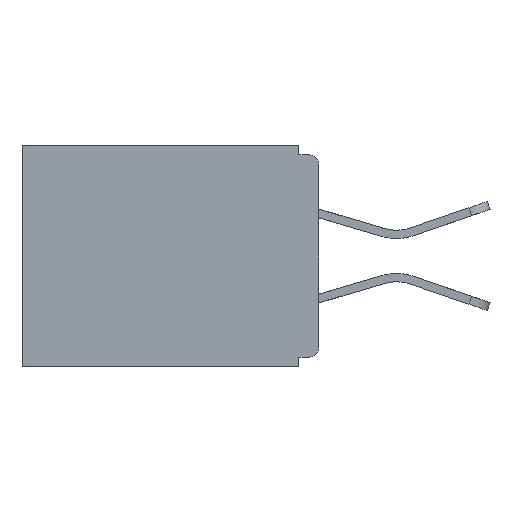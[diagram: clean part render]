
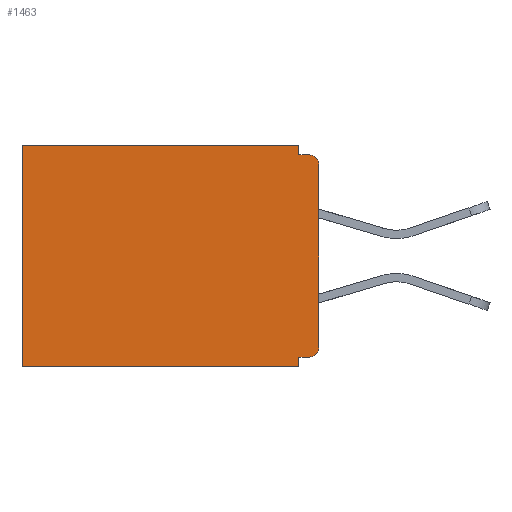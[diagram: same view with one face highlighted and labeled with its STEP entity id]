
A CAD part, left-side view. The second image highlights one B-rep face of the part: STEP entity #1463.
In plain terms, the highlighted planar face has unit normal (-1, 0, 0).
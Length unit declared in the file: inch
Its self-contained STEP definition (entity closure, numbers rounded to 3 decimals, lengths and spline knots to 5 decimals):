
#153 = EDGE_CURVE ( 'NONE', #609, #22547, #23457, .T. ) ;
#447 = VERTEX_POINT ( 'NONE', #2429 ) ;
#609 = VERTEX_POINT ( 'NONE', #21421 ) ;
#744 = ORIENTED_EDGE ( 'NONE', *, *, #2330, .F. ) ;
#1193 = VECTOR ( 'NONE', #18090, 39.37008 ) ;
#1463 = ADVANCED_FACE ( 'NONE', ( #21508 ), #23409, .F. ) ;
#1620 = EDGE_CURVE ( 'NONE', #26371, #25708, #7980, .T. ) ;
#2048 = DIRECTION ( 'NONE',  ( 0., 1., 0. ) ) ;
#2223 = DIRECTION ( 'NONE',  ( 0., 1., 0. ) ) ;
#2301 = DIRECTION ( 'NONE',  ( 0., 0., -1. ) ) ;
#2330 = EDGE_CURVE ( 'NONE', #10752, #23566, #10730, .T. ) ;
#2429 = CARTESIAN_POINT ( 'NONE',  ( 0.298, 0.46, -0.343 ) ) ;
#2965 = ORIENTED_EDGE ( 'NONE', *, *, #18822, .T. ) ;
#3306 = EDGE_CURVE ( 'NONE', #19995, #447, #14281, .T. ) ;
#3364 = CARTESIAN_POINT ( 'NONE',  ( 0.298, 0.031, -0.343 ) ) ;
#3389 = CARTESIAN_POINT ( 'NONE',  ( 0.298, 0.031, -0.015 ) ) ;
#3553 = DIRECTION ( 'NONE',  ( -1., 0., 0. ) ) ;
#3726 = CARTESIAN_POINT ( 'NONE',  ( 0.298, 0.015, -0.313 ) ) ;
#3766 = EDGE_CURVE ( 'NONE', #10752, #22547, #21981, .T. ) ;
#3982 = CARTESIAN_POINT ( 'NONE',  ( 0.298, 0.015, -0.328 ) ) ;
#4458 = ORIENTED_EDGE ( 'NONE', *, *, #12327, .F. ) ;
#4775 = VECTOR ( 'NONE', #24351, 39.37008 ) ;
#5101 = LINE ( 'NONE', #6859, #17348 ) ;
#5162 = CIRCLE ( 'NONE', #22326, 0.015 ) ;
#5208 = EDGE_CURVE ( 'NONE', #22347, #19995, #5101, .T. ) ;
#6859 = CARTESIAN_POINT ( 'NONE',  ( 0.298, 0., 0. ) ) ;
#7383 = ORIENTED_EDGE ( 'NONE', *, *, #3306, .T. ) ;
#7885 = VERTEX_POINT ( 'NONE', #18460 ) ;
#7980 = LINE ( 'NONE', #16224, #1193 ) ;
#8413 = ORIENTED_EDGE ( 'NONE', *, *, #19500, .F. ) ;
#8466 = VECTOR ( 'NONE', #9585, 39.37008 ) ;
#8694 = AXIS2_PLACEMENT_3D ( 'NONE', #3726, #3553, #20412 ) ;
#8833 = EDGE_LOOP ( 'NONE', ( #2965, #13243, #8413, #17820, #7383, #4458, #19652, #744, #18221, #15932 ) ) ;
#9081 = DIRECTION ( 'NONE',  ( 0., 0., -1. ) ) ;
#9177 = VECTOR ( 'NONE', #2301, 39.37008 ) ;
#9440 = DIRECTION ( 'NONE',  ( 0., 0., -1. ) ) ;
#9585 = DIRECTION ( 'NONE',  ( 0., 0., -1. ) ) ;
#10118 = CARTESIAN_POINT ( 'NONE',  ( 0.298, 0., -0.313 ) ) ;
#10321 = LINE ( 'NONE', #3364, #4775 ) ;
#10730 = LINE ( 'NONE', #18411, #11027 ) ;
#10752 = VERTEX_POINT ( 'NONE', #3982 ) ;
#11027 = VECTOR ( 'NONE', #2048, 39.37008 ) ;
#11192 = CARTESIAN_POINT ( 'NONE',  ( 0.298, 0., 0. ) ) ;
#11292 = DIRECTION ( 'NONE',  ( 0., 0., -1. ) ) ;
#12327 = EDGE_CURVE ( 'NONE', #7885, #447, #16733, .T. ) ;
#13243 = ORIENTED_EDGE ( 'NONE', *, *, #1620, .F. ) ;
#13726 = CARTESIAN_POINT ( 'NONE',  ( 0.298, 0.031, -0.328 ) ) ;
#14266 = EDGE_CURVE ( 'NONE', #23566, #7885, #21109, .T. ) ;
#14281 = LINE ( 'NONE', #25810, #8466 ) ;
#14482 = CARTESIAN_POINT ( 'NONE',  ( 0.298, 0.031, -0.343 ) ) ;
#14577 = AXIS2_PLACEMENT_3D ( 'NONE', #17080, #21433, #9081 ) ;
#14972 = CARTESIAN_POINT ( 'NONE',  ( 0.298, 0.015, -0.015 ) ) ;
#15847 = DIRECTION ( 'NONE',  ( -1., 0., 0. ) ) ;
#15932 = ORIENTED_EDGE ( 'NONE', *, *, #153, .F. ) ;
#16224 = CARTESIAN_POINT ( 'NONE',  ( 0.298, 0., -0.015 ) ) ;
#16419 = CARTESIAN_POINT ( 'NONE',  ( 0.298, 0.46, 0. ) ) ;
#16733 = LINE ( 'NONE', #21712, #23491 ) ;
#17080 = CARTESIAN_POINT ( 'NONE',  ( 0.298, 0., 0. ) ) ;
#17348 = VECTOR ( 'NONE', #2223, 39.37008 ) ;
#17749 = DIRECTION ( 'NONE',  ( 0., 1., 0. ) ) ;
#17820 = ORIENTED_EDGE ( 'NONE', *, *, #5208, .T. ) ;
#18090 = DIRECTION ( 'NONE',  ( 0., -1., 0. ) ) ;
#18221 = ORIENTED_EDGE ( 'NONE', *, *, #3766, .T. ) ;
#18411 = CARTESIAN_POINT ( 'NONE',  ( 0.298, 0., -0.328 ) ) ;
#18460 = CARTESIAN_POINT ( 'NONE',  ( 0.298, 0.031, -0.343 ) ) ;
#18625 = VECTOR ( 'NONE', #11292, 39.37008 ) ;
#18822 = EDGE_CURVE ( 'NONE', #609, #25708, #5162, .T. ) ;
#19500 = EDGE_CURVE ( 'NONE', #22347, #26371, #10321, .T. ) ;
#19652 = ORIENTED_EDGE ( 'NONE', *, *, #14266, .F. ) ;
#19945 = CARTESIAN_POINT ( 'NONE',  ( 0.298, 0.031, 0. ) ) ;
#19995 = VERTEX_POINT ( 'NONE', #16419 ) ;
#20412 = DIRECTION ( 'NONE',  ( 0., 0., -1. ) ) ;
#21109 = LINE ( 'NONE', #14482, #9177 ) ;
#21421 = CARTESIAN_POINT ( 'NONE',  ( 0.298, 0., -0.03 ) ) ;
#21433 = DIRECTION ( 'NONE',  ( 1., 0., 0. ) ) ;
#21508 = FACE_OUTER_BOUND ( 'NONE', #8833, .T. ) ;
#21712 = CARTESIAN_POINT ( 'NONE',  ( 0.298, 0., -0.343 ) ) ;
#21772 = CARTESIAN_POINT ( 'NONE',  ( 0.298, 0.015, -0.03 ) ) ;
#21981 = CIRCLE ( 'NONE', #8694, 0.015 ) ;
#22326 = AXIS2_PLACEMENT_3D ( 'NONE', #21772, #15847, #9440 ) ;
#22347 = VERTEX_POINT ( 'NONE', #19945 ) ;
#22547 = VERTEX_POINT ( 'NONE', #10118 ) ;
#23409 = PLANE ( 'NONE',  #14577 ) ;
#23457 = LINE ( 'NONE', #11192, #18625 ) ;
#23491 = VECTOR ( 'NONE', #17749, 39.37008 ) ;
#23566 = VERTEX_POINT ( 'NONE', #13726 ) ;
#24351 = DIRECTION ( 'NONE',  ( 0., 0., -1. ) ) ;
#25708 = VERTEX_POINT ( 'NONE', #14972 ) ;
#25810 = CARTESIAN_POINT ( 'NONE',  ( 0.298, 0.46, 0. ) ) ;
#26371 = VERTEX_POINT ( 'NONE', #3389 ) ;
